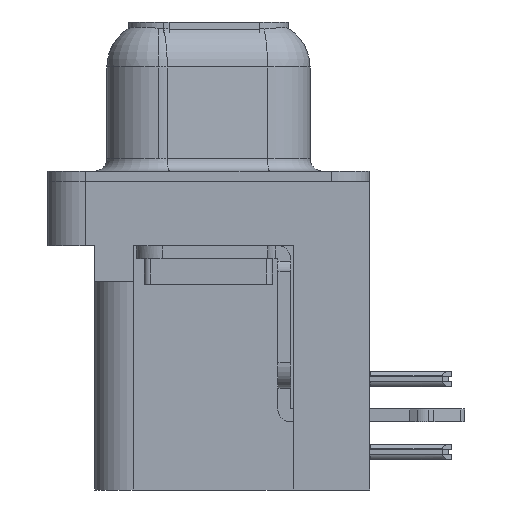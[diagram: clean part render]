
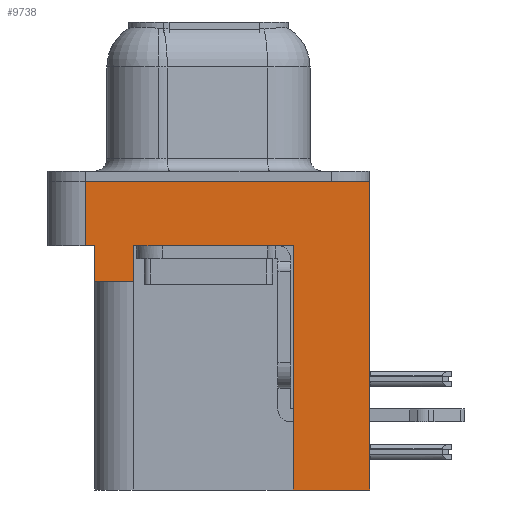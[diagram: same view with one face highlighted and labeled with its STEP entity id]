
A CAD part, left-side view. The second image highlights one B-rep face of the part: STEP entity #9738.
In plain terms, the highlighted planar face has unit normal (-1, 0, 0).
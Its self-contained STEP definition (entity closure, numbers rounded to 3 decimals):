
#592 = VERTEX_POINT ( 'NONE', #20304 ) ;
#1140 = DIRECTION ( 'NONE',  ( 0., 0., 1. ) ) ;
#2585 = ORIENTED_EDGE ( 'NONE', *, *, #13646, .F. ) ;
#2613 = EDGE_CURVE ( 'NONE', #28469, #18962, #7434, .T. ) ;
#2712 = EDGE_CURVE ( 'NONE', #18962, #20167, #27359, .T. ) ;
#3417 = DIRECTION ( 'NONE',  ( 0., 0., 1. ) ) ;
#3653 = VECTOR ( 'NONE', #14618, 1000. ) ;
#3657 = DIRECTION ( 'NONE',  ( 0., 0., 1. ) ) ;
#3673 = LINE ( 'NONE', #14247, #3653 ) ;
#4045 = LINE ( 'NONE', #20864, #11142 ) ;
#4129 = EDGE_CURVE ( 'NONE', #592, #10829, #29405, .T. ) ;
#4204 = CARTESIAN_POINT ( 'NONE',  ( -3., -6.275, 0. ) ) ;
#5119 = EDGE_CURVE ( 'NONE', #8441, #592, #27567, .T. ) ;
#5582 = EDGE_CURVE ( 'NONE', #17976, #10829, #29303, .T. ) ;
#5928 = VECTOR ( 'NONE', #20709, 1000. ) ;
#5980 = VECTOR ( 'NONE', #3417, 1000. ) ;
#6416 = EDGE_LOOP ( 'NONE', ( #13091, #14753, #28194, #21540, #28371, #25513, #9428, #24415, #2585, #9727 ) ) ;
#7418 = EDGE_CURVE ( 'NONE', #9317, #24093, #15894, .T. ) ;
#7434 = LINE ( 'NONE', #28992, #23053 ) ;
#7515 = DIRECTION ( 'NONE',  ( 0., 1., 0. ) ) ;
#7791 = CARTESIAN_POINT ( 'NONE',  ( -3., -6.275, -2.5 ) ) ;
#8309 = AXIS2_PLACEMENT_3D ( 'NONE', #23333, #27942, #1140 ) ;
#8376 = VECTOR ( 'NONE', #10637, 1000. ) ;
#8441 = VERTEX_POINT ( 'NONE', #12488 ) ;
#8583 = CARTESIAN_POINT ( 'NONE',  ( -3., 4.425, -3.9 ) ) ;
#9055 = VECTOR ( 'NONE', #3657, 1000. ) ;
#9317 = VERTEX_POINT ( 'NONE', #21161 ) ;
#9428 = ORIENTED_EDGE ( 'NONE', *, *, #7418, .T. ) ;
#9727 = ORIENTED_EDGE ( 'NONE', *, *, #5582, .T. ) ;
#9738 = ADVANCED_FACE ( 'NONE', ( #28170 ), #25448, .T. ) ;
#10637 = DIRECTION ( 'NONE',  ( 0., 0., 1. ) ) ;
#10829 = VERTEX_POINT ( 'NONE', #4204 ) ;
#11142 = VECTOR ( 'NONE', #7515, 1000. ) ;
#11390 = CARTESIAN_POINT ( 'NONE',  ( -3., -6.275, -2.5 ) ) ;
#11648 = VECTOR ( 'NONE', #19221, 1000. ) ;
#12098 = EDGE_CURVE ( 'NONE', #28469, #9317, #27707, .T. ) ;
#12488 = CARTESIAN_POINT ( 'NONE',  ( -3., 4.775, -2.5 ) ) ;
#12667 = CARTESIAN_POINT ( 'NONE',  ( -3., -3.295, -2.5 ) ) ;
#13091 = ORIENTED_EDGE ( 'NONE', *, *, #4129, .F. ) ;
#13428 = DIRECTION ( 'NONE',  ( 0., 0., 1. ) ) ;
#13646 = EDGE_CURVE ( 'NONE', #17976, #24077, #4045, .T. ) ;
#14247 = CARTESIAN_POINT ( 'NONE',  ( -3., -6.275, -2.5 ) ) ;
#14248 = EDGE_CURVE ( 'NONE', #24077, #24093, #24079, .T. ) ;
#14618 = DIRECTION ( 'NONE',  ( 0., -1., 0. ) ) ;
#14746 = CARTESIAN_POINT ( 'NONE',  ( -3., -3.295, -12. ) ) ;
#14753 = ORIENTED_EDGE ( 'NONE', *, *, #5119, .F. ) ;
#14851 = CARTESIAN_POINT ( 'NONE',  ( -3., 2.895, -3.9 ) ) ;
#14915 = VECTOR ( 'NONE', #13428, 1000. ) ;
#15494 = DIRECTION ( 'NONE',  ( 0., 0., 1. ) ) ;
#15894 = LINE ( 'NONE', #11390, #5928 ) ;
#16332 = CARTESIAN_POINT ( 'NONE',  ( -3., 2.895, -3.9 ) ) ;
#17060 = CARTESIAN_POINT ( 'NONE',  ( -3., -6.275, 0. ) ) ;
#17976 = VERTEX_POINT ( 'NONE', #22764 ) ;
#18962 = VERTEX_POINT ( 'NONE', #8583 ) ;
#19221 = DIRECTION ( 'NONE',  ( 0., -1., 0. ) ) ;
#19794 = CARTESIAN_POINT ( 'NONE',  ( -3., 4.775, -2.5 ) ) ;
#20167 = VERTEX_POINT ( 'NONE', #25889 ) ;
#20304 = CARTESIAN_POINT ( 'NONE',  ( -3., 4.775, 0. ) ) ;
#20709 = DIRECTION ( 'NONE',  ( 0., -1., 0. ) ) ;
#20864 = CARTESIAN_POINT ( 'NONE',  ( -3., -3.295, -12. ) ) ;
#21161 = CARTESIAN_POINT ( 'NONE',  ( -3., 2.895, -2.5 ) ) ;
#21276 = CARTESIAN_POINT ( 'NONE',  ( -3., -3.295, -12. ) ) ;
#21540 = ORIENTED_EDGE ( 'NONE', *, *, #2712, .F. ) ;
#21648 = VECTOR ( 'NONE', #15494, 1000. ) ;
#22433 = CARTESIAN_POINT ( 'NONE',  ( -3., 4.425, -3.9 ) ) ;
#22764 = CARTESIAN_POINT ( 'NONE',  ( -3., -6.275, -12. ) ) ;
#23053 = VECTOR ( 'NONE', #24022, 1000. ) ;
#23333 = CARTESIAN_POINT ( 'NONE',  ( -3., -6.275, -2.5 ) ) ;
#24022 = DIRECTION ( 'NONE',  ( 0., 1., 0. ) ) ;
#24077 = VERTEX_POINT ( 'NONE', #14746 ) ;
#24079 = LINE ( 'NONE', #21276, #5980 ) ;
#24093 = VERTEX_POINT ( 'NONE', #12667 ) ;
#24415 = ORIENTED_EDGE ( 'NONE', *, *, #14248, .F. ) ;
#25448 = PLANE ( 'NONE',  #8309 ) ;
#25513 = ORIENTED_EDGE ( 'NONE', *, *, #12098, .T. ) ;
#25889 = CARTESIAN_POINT ( 'NONE',  ( -3., 4.425, -2.5 ) ) ;
#27359 = LINE ( 'NONE', #22433, #14915 ) ;
#27567 = LINE ( 'NONE', #19794, #8376 ) ;
#27707 = LINE ( 'NONE', #16332, #21648 ) ;
#27942 = DIRECTION ( 'NONE',  ( -1., 0., 0. ) ) ;
#28170 = FACE_OUTER_BOUND ( 'NONE', #6416, .T. ) ;
#28194 = ORIENTED_EDGE ( 'NONE', *, *, #29127, .T. ) ;
#28371 = ORIENTED_EDGE ( 'NONE', *, *, #2613, .F. ) ;
#28469 = VERTEX_POINT ( 'NONE', #14851 ) ;
#28992 = CARTESIAN_POINT ( 'NONE',  ( -3., 4.425, -3.9 ) ) ;
#29127 = EDGE_CURVE ( 'NONE', #8441, #20167, #3673, .T. ) ;
#29303 = LINE ( 'NONE', #7791, #9055 ) ;
#29405 = LINE ( 'NONE', #17060, #11648 ) ;
